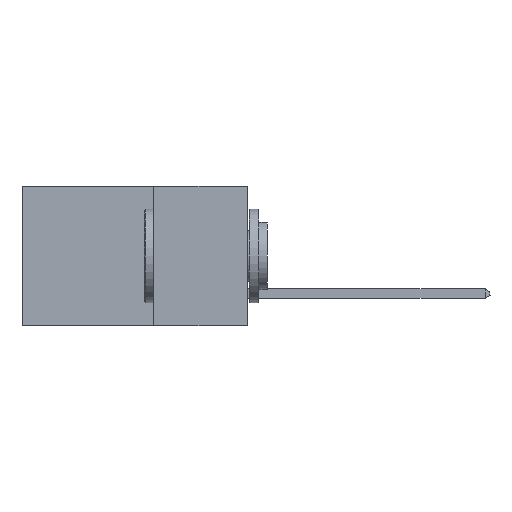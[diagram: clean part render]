
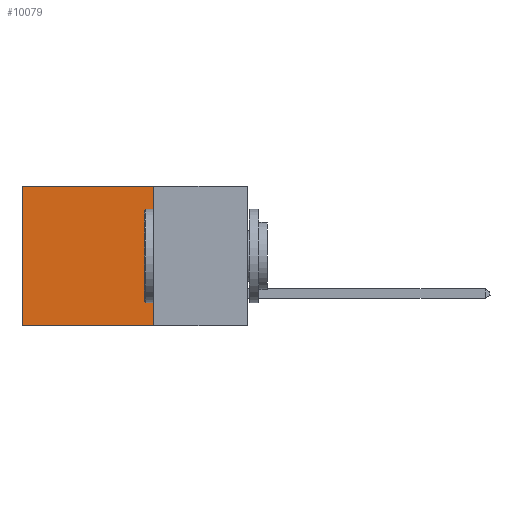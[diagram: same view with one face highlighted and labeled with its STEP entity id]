
A CAD part, left-side view. The second image highlights one B-rep face of the part: STEP entity #10079.
In plain terms, the highlighted planar face has unit normal (-1, 0, 0).
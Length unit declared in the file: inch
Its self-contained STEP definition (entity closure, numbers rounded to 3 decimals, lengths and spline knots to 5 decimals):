
#340 = CARTESIAN_POINT ( 'NONE',  ( 0.298, 0.25, 0. ) ) ;
#511 = VECTOR ( 'NONE', #9169, 39.37008 ) ;
#630 = EDGE_CURVE ( 'NONE', #2994, #9296, #11918, .T. ) ;
#869 = LINE ( 'NONE', #9020, #511 ) ;
#1160 = EDGE_CURVE ( 'NONE', #4625, #1222, #869, .T. ) ;
#1222 = VERTEX_POINT ( 'NONE', #9934 ) ;
#1506 = DIRECTION ( 'NONE',  ( 0., 1., 0. ) ) ;
#2574 = EDGE_CURVE ( 'NONE', #9296, #1222, #8352, .T. ) ;
#2665 = FACE_OUTER_BOUND ( 'NONE', #13665, .T. ) ;
#2994 = VERTEX_POINT ( 'NONE', #11503 ) ;
#3616 = ORIENTED_EDGE ( 'NONE', *, *, #5829, .T. ) ;
#3682 = VECTOR ( 'NONE', #1506, 39.37008 ) ;
#4625 = VERTEX_POINT ( 'NONE', #12236 ) ;
#4704 = LINE ( 'NONE', #340, #3682 ) ;
#4708 = CARTESIAN_POINT ( 'NONE',  ( 0.298, 0.25, -0.37 ) ) ;
#5829 = EDGE_CURVE ( 'NONE', #2994, #4625, #4704, .T. ) ;
#7348 = PLANE ( 'NONE',  #11404 ) ;
#8230 = CARTESIAN_POINT ( 'NONE',  ( 0.298, 0.25, -0.37 ) ) ;
#8302 = DIRECTION ( 'NONE',  ( 0., 0., -1. ) ) ;
#8352 = LINE ( 'NONE', #8230, #12936 ) ;
#8401 = CARTESIAN_POINT ( 'NONE',  ( 0.298, 0.25, 0. ) ) ;
#8463 = DIRECTION ( 'NONE',  ( 0., 0., -1. ) ) ;
#9020 = CARTESIAN_POINT ( 'NONE',  ( 0.298, 0.6, 0. ) ) ;
#9169 = DIRECTION ( 'NONE',  ( 0., 0., -1. ) ) ;
#9243 = ORIENTED_EDGE ( 'NONE', *, *, #630, .F. ) ;
#9296 = VERTEX_POINT ( 'NONE', #4708 ) ;
#9634 = CARTESIAN_POINT ( 'NONE',  ( 0.298, 0.25, 0. ) ) ;
#9716 = ORIENTED_EDGE ( 'NONE', *, *, #1160, .T. ) ;
#9934 = CARTESIAN_POINT ( 'NONE',  ( 0.298, 0.6, -0.37 ) ) ;
#10079 = ADVANCED_FACE ( 'NONE', ( #2665 ), #7348, .F. ) ;
#10472 = DIRECTION ( 'NONE',  ( 0., 1., 0. ) ) ;
#10507 = DIRECTION ( 'NONE',  ( 1., 0., 0. ) ) ;
#11404 = AXIS2_PLACEMENT_3D ( 'NONE', #8401, #10507, #8302 ) ;
#11456 = ORIENTED_EDGE ( 'NONE', *, *, #2574, .F. ) ;
#11503 = CARTESIAN_POINT ( 'NONE',  ( 0.298, 0.25, 0. ) ) ;
#11918 = LINE ( 'NONE', #9634, #12436 ) ;
#12236 = CARTESIAN_POINT ( 'NONE',  ( 0.298, 0.6, 0. ) ) ;
#12436 = VECTOR ( 'NONE', #8463, 39.37008 ) ;
#12936 = VECTOR ( 'NONE', #10472, 39.37008 ) ;
#13665 = EDGE_LOOP ( 'NONE', ( #9716, #11456, #9243, #3616 ) ) ;
